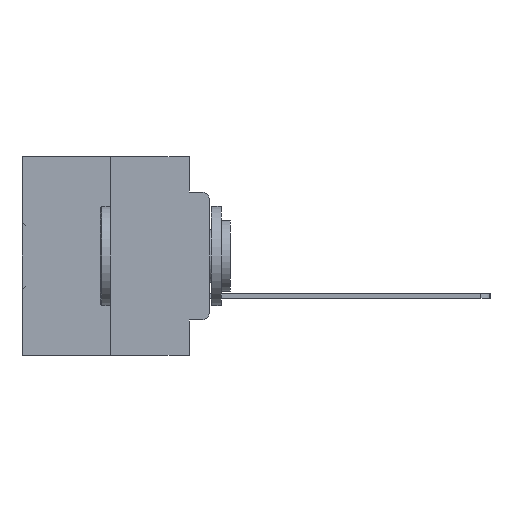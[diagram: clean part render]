
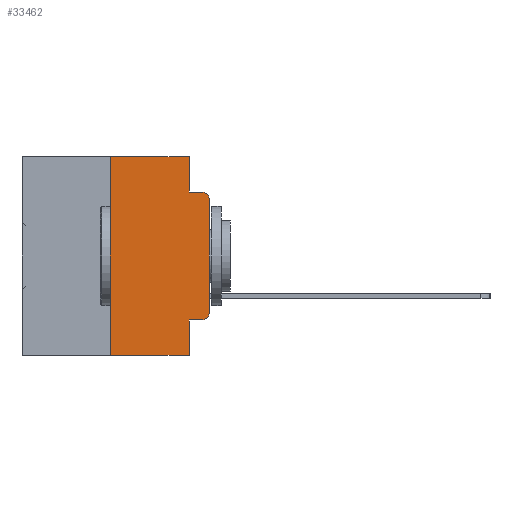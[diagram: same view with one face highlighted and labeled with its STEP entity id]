
A CAD part, left-side view. The second image highlights one B-rep face of the part: STEP entity #33462.
In plain terms, the highlighted planar face has unit normal (-1, 0, 0).
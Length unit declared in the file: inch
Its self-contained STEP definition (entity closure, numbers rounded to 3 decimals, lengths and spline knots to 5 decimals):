
#225 = CARTESIAN_POINT ( 'NONE',  ( 0., 0., -0.1085 ) ) ;
#365 = CARTESIAN_POINT ( 'NONE',  ( 0., 0.25, -0.5 ) ) ;
#502 = VERTEX_POINT ( 'NONE', #27653 ) ;
#682 = CARTESIAN_POINT ( 'NONE',  ( 0., 0.051, -0.0885 ) ) ;
#1995 = ORIENTED_EDGE ( 'NONE', *, *, #30538, .T. ) ;
#2046 = VECTOR ( 'NONE', #33139, 39.37008 ) ;
#3524 = DIRECTION ( 'NONE',  ( 1., 0., 0. ) ) ;
#3619 = CARTESIAN_POINT ( 'NONE',  ( 0., 0.02, -0.0885 ) ) ;
#4279 = ORIENTED_EDGE ( 'NONE', *, *, #33989, .F. ) ;
#4577 = LINE ( 'NONE', #14314, #32919 ) ;
#4861 = CARTESIAN_POINT ( 'NONE',  ( 0., 0.051, 0. ) ) ;
#5548 = VERTEX_POINT ( 'NONE', #24131 ) ;
#5760 = LINE ( 'NONE', #32862, #33268 ) ;
#6043 = VERTEX_POINT ( 'NONE', #31322 ) ;
#6236 = LINE ( 'NONE', #682, #19760 ) ;
#6240 = ORIENTED_EDGE ( 'NONE', *, *, #23198, .F. ) ;
#7017 = EDGE_CURVE ( 'NONE', #33369, #6043, #4577, .T. ) ;
#7109 = CARTESIAN_POINT ( 'NONE',  ( 0., 0., 0. ) ) ;
#7321 = FACE_OUTER_BOUND ( 'NONE', #16784, .T. ) ;
#7811 = VERTEX_POINT ( 'NONE', #31106 ) ;
#8979 = VECTOR ( 'NONE', #18722, 39.37008 ) ;
#9261 = LINE ( 'NONE', #12123, #2046 ) ;
#10087 = ORIENTED_EDGE ( 'NONE', *, *, #14805, .F. ) ;
#10177 = CIRCLE ( 'NONE', #15655, 0.02 ) ;
#10605 = CARTESIAN_POINT ( 'NONE',  ( 0., 0.473, -0.5 ) ) ;
#10691 = ORIENTED_EDGE ( 'NONE', *, *, #18611, .T. ) ;
#11739 = DIRECTION ( 'NONE',  ( -1., 0., 0. ) ) ;
#12123 = CARTESIAN_POINT ( 'NONE',  ( 0., 0.473, 0. ) ) ;
#12206 = CARTESIAN_POINT ( 'NONE',  ( 0., 0., -0.3915 ) ) ;
#13881 = DIRECTION ( 'NONE',  ( -1., 0., 0. ) ) ;
#14014 = AXIS2_PLACEMENT_3D ( 'NONE', #27617, #11739, #30274 ) ;
#14314 = CARTESIAN_POINT ( 'NONE',  ( 0., 0.25, 0. ) ) ;
#14437 = DIRECTION ( 'NONE',  ( 0., 0., -1. ) ) ;
#14805 = EDGE_CURVE ( 'NONE', #34332, #28819, #6236, .T. ) ;
#15469 = EDGE_CURVE ( 'NONE', #5548, #34332, #5760, .T. ) ;
#15655 = AXIS2_PLACEMENT_3D ( 'NONE', #29735, #13881, #32331 ) ;
#16562 = LINE ( 'NONE', #10605, #22764 ) ;
#16784 = EDGE_LOOP ( 'NONE', ( #21796, #1995, #10087, #25108, #6240, #27576, #10691, #4279, #28152, #17036 ) ) ;
#17036 = ORIENTED_EDGE ( 'NONE', *, *, #27153, .T. ) ;
#17050 = CARTESIAN_POINT ( 'NONE',  ( 0., 0.051, -0.0885 ) ) ;
#17942 = AXIS2_PLACEMENT_3D ( 'NONE', #27554, #3524, #22369 ) ;
#18004 = DIRECTION ( 'NONE',  ( 0., 0., 1. ) ) ;
#18611 = EDGE_CURVE ( 'NONE', #33369, #31854, #16562, .T. ) ;
#18722 = DIRECTION ( 'NONE',  ( 0., -1., 0. ) ) ;
#19588 = DIRECTION ( 'NONE',  ( 0., -1., 0. ) ) ;
#19740 = PLANE ( 'NONE',  #17942 ) ;
#19760 = VECTOR ( 'NONE', #19588, 39.37008 ) ;
#20307 = CARTESIAN_POINT ( 'NONE',  ( 0., 0.051, -0.5 ) ) ;
#21796 = ORIENTED_EDGE ( 'NONE', *, *, #33899, .T. ) ;
#22369 = DIRECTION ( 'NONE',  ( 0., 0., -1. ) ) ;
#22764 = VECTOR ( 'NONE', #31795, 39.37008 ) ;
#23198 = EDGE_CURVE ( 'NONE', #6043, #5548, #9261, .T. ) ;
#23650 = DIRECTION ( 'NONE',  ( 0., 0., -1. ) ) ;
#24131 = CARTESIAN_POINT ( 'NONE',  ( 0., 0.051, 0. ) ) ;
#25108 = ORIENTED_EDGE ( 'NONE', *, *, #15469, .F. ) ;
#25321 = VECTOR ( 'NONE', #23650, 39.37008 ) ;
#25838 = CIRCLE ( 'NONE', #14014, 0.02 ) ;
#27153 = EDGE_CURVE ( 'NONE', #502, #27275, #25838, .T. ) ;
#27275 = VERTEX_POINT ( 'NONE', #12206 ) ;
#27554 = CARTESIAN_POINT ( 'NONE',  ( 0., 0.473, 0. ) ) ;
#27576 = ORIENTED_EDGE ( 'NONE', *, *, #7017, .F. ) ;
#27617 = CARTESIAN_POINT ( 'NONE',  ( 0., 0.02, -0.3915 ) ) ;
#27653 = CARTESIAN_POINT ( 'NONE',  ( 0., 0.02, -0.4115 ) ) ;
#27786 = VECTOR ( 'NONE', #18004, 39.37008 ) ;
#28152 = ORIENTED_EDGE ( 'NONE', *, *, #29166, .T. ) ;
#28621 = LINE ( 'NONE', #7109, #27786 ) ;
#28658 = VERTEX_POINT ( 'NONE', #225 ) ;
#28819 = VERTEX_POINT ( 'NONE', #3619 ) ;
#29166 = EDGE_CURVE ( 'NONE', #7811, #502, #29410, .T. ) ;
#29410 = LINE ( 'NONE', #34499, #8979 ) ;
#29735 = CARTESIAN_POINT ( 'NONE',  ( 0., 0.02, -0.1085 ) ) ;
#30274 = DIRECTION ( 'NONE',  ( 0., 0., -1. ) ) ;
#30538 = EDGE_CURVE ( 'NONE', #28658, #28819, #10177, .T. ) ;
#31106 = CARTESIAN_POINT ( 'NONE',  ( 0., 0.051, -0.4115 ) ) ;
#31322 = CARTESIAN_POINT ( 'NONE',  ( 0., 0.25, 0. ) ) ;
#31795 = DIRECTION ( 'NONE',  ( 0., -1., 0. ) ) ;
#31854 = VERTEX_POINT ( 'NONE', #20307 ) ;
#32279 = LINE ( 'NONE', #4861, #25321 ) ;
#32331 = DIRECTION ( 'NONE',  ( 0., 0., -1. ) ) ;
#32747 = DIRECTION ( 'NONE',  ( 0., 0., 1. ) ) ;
#32862 = CARTESIAN_POINT ( 'NONE',  ( 0., 0.051, 0. ) ) ;
#32919 = VECTOR ( 'NONE', #32747, 39.37008 ) ;
#33139 = DIRECTION ( 'NONE',  ( 0., -1., 0. ) ) ;
#33268 = VECTOR ( 'NONE', #14437, 39.37008 ) ;
#33369 = VERTEX_POINT ( 'NONE', #365 ) ;
#33462 = ADVANCED_FACE ( 'NONE', ( #7321 ), #19740, .F. ) ;
#33899 = EDGE_CURVE ( 'NONE', #27275, #28658, #28621, .T. ) ;
#33989 = EDGE_CURVE ( 'NONE', #7811, #31854, #32279, .T. ) ;
#34332 = VERTEX_POINT ( 'NONE', #17050 ) ;
#34499 = CARTESIAN_POINT ( 'NONE',  ( 0., 0.051, -0.4115 ) ) ;
